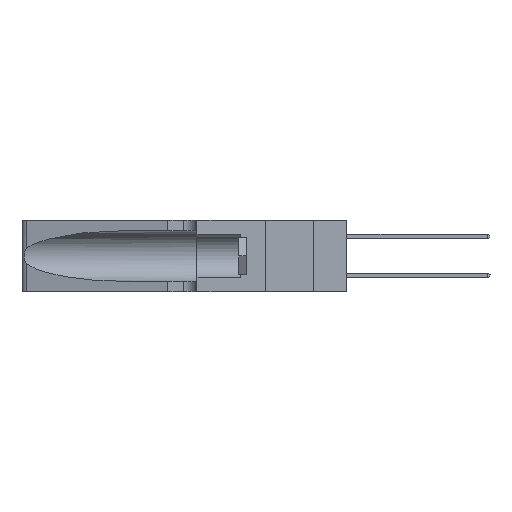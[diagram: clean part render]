
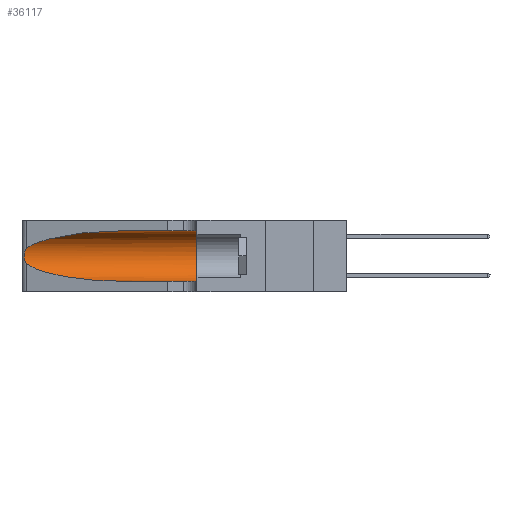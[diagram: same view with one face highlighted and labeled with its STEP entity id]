
A CAD part, left-side view. The second image highlights one B-rep face of the part: STEP entity #36117.
In plain terms, the highlighted cylindrical face has radius 3.308 mm (diameter 6.617 mm), a partial arc.
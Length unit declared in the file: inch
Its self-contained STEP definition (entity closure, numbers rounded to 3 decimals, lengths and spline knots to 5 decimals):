
#97 = EDGE_CURVE ( 'NONE', #19778, #24163, #12762, .T. ) ;
#454 = CARTESIAN_POINT ( 'NONE',  ( 0.25787, 1.23484, 0.2124 ) ) ;
#528 = EDGE_CURVE ( 'NONE', #37291, #10266, #10215, .T. ) ;
#1411 = EDGE_CURVE ( 'NONE', #2716, #10266, #22525, .T. ) ;
#2328 =( BOUNDED_CURVE ( )  B_SPLINE_CURVE ( 3, ( #42541, #12626, #31491, #8965 ),
 .UNSPECIFIED., .F., .F. ) 
 B_SPLINE_CURVE_WITH_KNOTS ( ( 4, 4 ),
 ( 3.44316, 4.71239 ),
 .UNSPECIFIED. ) 
 CURVE ( )  GEOMETRIC_REPRESENTATION_ITEM ( )  RATIONAL_B_SPLINE_CURVE ( ( 1., 0.87, 0.87, 1. ) ) 
 REPRESENTATION_ITEM ( '' )  );
#2716 = VERTEX_POINT ( 'NONE', #41531 ) ;
#2974 = CARTESIAN_POINT ( 'NONE',  ( 0.1305, 0.72297, 0.31525 ) ) ;
#4316 = CARTESIAN_POINT ( 'NONE',  ( 0.26018, 1.23835, 0.19895 ) ) ;
#7942 = EDGE_CURVE ( 'NONE', #23928, #37291, #48664, .T. ) ;
#8004 = CARTESIAN_POINT ( 'NONE',  ( 0.25487, 1.22718, 0.22369 ) ) ;
#8175 = CARTESIAN_POINT ( 'NONE',  ( 0.26075, 1.23896, 0.178 ) ) ;
#8258 = CARTESIAN_POINT ( 'NONE',  ( 0.1305, 1.61858, 0.185 ) ) ;
#8965 = CARTESIAN_POINT ( 'NONE',  ( 0.1305, 0.72297, 0.05475 ) ) ;
#9381 = CARTESIAN_POINT ( 'NONE',  ( 0.18966, 0.96281, 0.31525 ) ) ;
#10215 = CIRCLE ( 'NONE', #43871, 0.13025 ) ;
#10266 = VERTEX_POINT ( 'NONE', #36965 ) ;
#11109 = DIRECTION ( 'NONE',  ( 0., 1., 0. ) ) ;
#12003 = CARTESIAN_POINT ( 'NONE',  ( 0.25856, 1.23593, 0.16098 ) ) ;
#12444 = CYLINDRICAL_SURFACE ( 'NONE', #18903, 0.13025 ) ;
#12626 = CARTESIAN_POINT ( 'NONE',  ( 0.2373, 1.15595, 0.08982 ) ) ;
#12762 = B_SPLINE_CURVE_WITH_KNOTS ( 'NONE', 3,
 ( #8004, #19460, #23212, #454, #26958, #4316, #30734, #8175, #34530, #12003, #38212, #15837, #41949, #19622 ),
 .UNSPECIFIED., .F., .F.,
 ( 4, 2, 2, 2, 2, 2, 4 ),
 ( 0., 0.00027, 0.00053, 0.00107, 0.0016, 0.00187, 0.00214 ),
 .UNSPECIFIED. ) ;
#13216 = CARTESIAN_POINT ( 'NONE',  ( 0.2373, 1.15595, 0.28018 ) ) ;
#14547 = ORIENTED_EDGE ( 'NONE', *, *, #1411, .T. ) ;
#14832 = EDGE_CURVE ( 'NONE', #24163, #2716, #2328, .T. ) ;
#15837 = CARTESIAN_POINT ( 'NONE',  ( 0.25639, 1.23186, 0.15144 ) ) ;
#18903 = AXIS2_PLACEMENT_3D ( 'NONE', #8258, #34591, #30800 ) ;
#19247 = CARTESIAN_POINT ( 'NONE',  ( 0.25487, 1.22718, 0.22369 ) ) ;
#19460 = CARTESIAN_POINT ( 'NONE',  ( 0.25555, 1.22994, 0.2215 ) ) ;
#19622 = CARTESIAN_POINT ( 'NONE',  ( 0.25487, 1.22718, 0.14631 ) ) ;
#19636 = CARTESIAN_POINT ( 'NONE',  ( 0.1305, 1.61858, 0.31525 ) ) ;
#19778 = VERTEX_POINT ( 'NONE', #19247 ) ;
#22525 = LINE ( 'NONE', #45598, #42367 ) ;
#23212 = CARTESIAN_POINT ( 'NONE',  ( 0.25639, 1.23184, 0.21858 ) ) ;
#23464 = ORIENTED_EDGE ( 'NONE', *, *, #7942, .F. ) ;
#23740 = EDGE_CURVE ( 'NONE', #23928, #19778, #25097, .T. ) ;
#23928 = VERTEX_POINT ( 'NONE', #2974 ) ;
#24163 = VERTEX_POINT ( 'NONE', #30724 ) ;
#25097 =( BOUNDED_CURVE ( )  B_SPLINE_CURVE ( 3, ( #42965, #9381, #13216, #39379 ),
 .UNSPECIFIED., .F., .F. ) 
 B_SPLINE_CURVE_WITH_KNOTS ( ( 4, 4 ),
 ( 1.5708, 2.84003 ),
 .UNSPECIFIED. ) 
 CURVE ( )  GEOMETRIC_REPRESENTATION_ITEM ( )  RATIONAL_B_SPLINE_CURVE ( ( 1., 0.87, 0.87, 1. ) ) 
 REPRESENTATION_ITEM ( '' )  );
#26958 = CARTESIAN_POINT ( 'NONE',  ( 0.25854, 1.2359, 0.20912 ) ) ;
#26985 = DIRECTION ( 'NONE',  ( 0., -1., 0. ) ) ;
#30724 = CARTESIAN_POINT ( 'NONE',  ( 0.25487, 1.22718, 0.14631 ) ) ;
#30734 = CARTESIAN_POINT ( 'NONE',  ( 0.26075, 1.23896, 0.19203 ) ) ;
#30800 = DIRECTION ( 'NONE',  ( 0., 0., -1. ) ) ;
#30970 = ORIENTED_EDGE ( 'NONE', *, *, #14832, .T. ) ;
#31491 = CARTESIAN_POINT ( 'NONE',  ( 0.18966, 0.96281, 0.05475 ) ) ;
#33618 = CARTESIAN_POINT ( 'NONE',  ( 0.1305, 0.35, 0.185 ) ) ;
#33947 = ORIENTED_EDGE ( 'NONE', *, *, #528, .F. ) ;
#34530 = CARTESIAN_POINT ( 'NONE',  ( 0.26017, 1.23833, 0.17102 ) ) ;
#34591 = DIRECTION ( 'NONE',  ( 0., -1., 0. ) ) ;
#36117 = ADVANCED_FACE ( 'NONE', ( #42299 ), #12444, .F. ) ;
#36965 = CARTESIAN_POINT ( 'NONE',  ( 0.1305, 0.35, 0.05475 ) ) ;
#37114 = ORIENTED_EDGE ( 'NONE', *, *, #97, .T. ) ;
#37291 = VERTEX_POINT ( 'NONE', #41921 ) ;
#37337 = DIRECTION ( 'NONE',  ( 0., 0., 1. ) ) ;
#38212 = CARTESIAN_POINT ( 'NONE',  ( 0.25789, 1.23486, 0.15765 ) ) ;
#38760 = VECTOR ( 'NONE', #41971, 39.37008 ) ;
#39379 = CARTESIAN_POINT ( 'NONE',  ( 0.25487, 1.22718, 0.22369 ) ) ;
#40873 = EDGE_LOOP ( 'NONE', ( #41954, #37114, #30970, #14547, #33947, #23464 ) ) ;
#41531 = CARTESIAN_POINT ( 'NONE',  ( 0.1305, 0.72297, 0.05475 ) ) ;
#41921 = CARTESIAN_POINT ( 'NONE',  ( 0.1305, 0.35, 0.31525 ) ) ;
#41949 = CARTESIAN_POINT ( 'NONE',  ( 0.25555, 1.22993, 0.14849 ) ) ;
#41954 = ORIENTED_EDGE ( 'NONE', *, *, #23740, .T. ) ;
#41971 = DIRECTION ( 'NONE',  ( 0., -1., 0. ) ) ;
#42299 = FACE_OUTER_BOUND ( 'NONE', #40873, .T. ) ;
#42367 = VECTOR ( 'NONE', #26985, 39.37008 ) ;
#42541 = CARTESIAN_POINT ( 'NONE',  ( 0.25487, 1.22718, 0.14631 ) ) ;
#42965 = CARTESIAN_POINT ( 'NONE',  ( 0.1305, 0.72297, 0.31525 ) ) ;
#43871 = AXIS2_PLACEMENT_3D ( 'NONE', #33618, #11109, #37337 ) ;
#45598 = CARTESIAN_POINT ( 'NONE',  ( 0.1305, 1.61858, 0.05475 ) ) ;
#48664 = LINE ( 'NONE', #19636, #38760 ) ;
